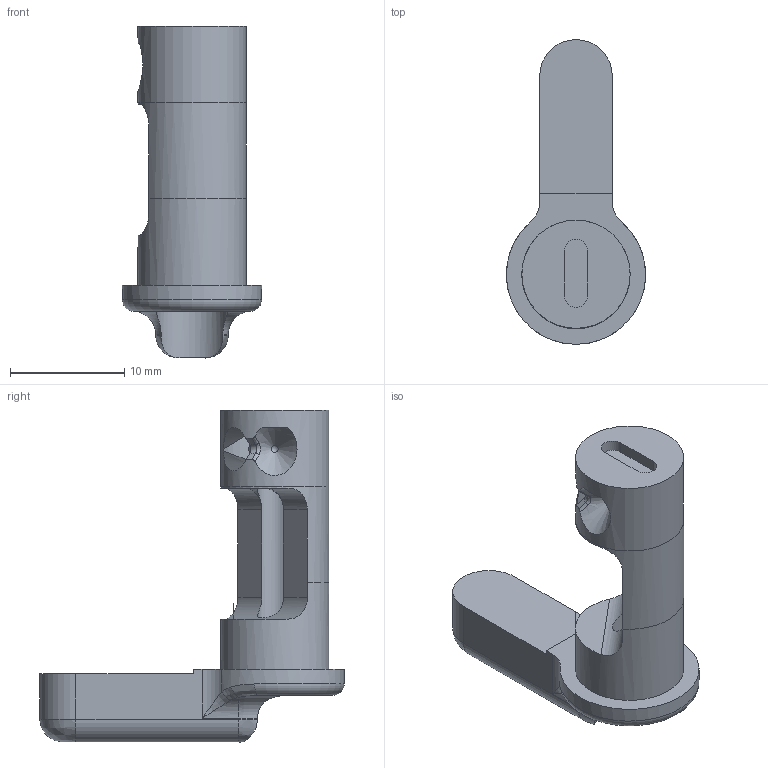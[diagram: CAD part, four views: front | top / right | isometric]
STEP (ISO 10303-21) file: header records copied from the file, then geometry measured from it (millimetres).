
FILE_DESCRIPTION(/* description */ (''),/* implementation_level */ '2;1');
FILE_NAME(/* name */ 'Fire Selector Lever.step',/* time_stamp */ '2022-05-12T09:38:32-06:00',/* author */ (''),/* organization */ (''),/* preprocessor_version */ 'ST-DEVELOPER v18.1',/* originating_system */ 'Autodesk Translation Framework v10.10.0.1391',/* authorisation */ '');
FILE_SCHEMA (('AUTOMOTIVE_DESIGN { 1 0 10303 214 3 1 1 }'));
Length unit declared in the file: millimetre
Products named in the file (1): Fire Selector Lever and drum.
Bounding box: 12.19 x 26.67 x 29.06 mm (x, y, z)
Volume: 1920.6 mm3; surface area: 1544.1 mm2
Topology: 1 solids, 2 shells, 79 faces, 210 edges, 135 vertices
Faces by surface type: plane 29, cylinder 26, bspline 14, cone 4, torus 4, sphere 2
Full cylindrical faces by diameter (mm): 2.87 x1, 3 x1, 9.474 x3
Entity records: 3027 total; most frequent: CARTESIAN_POINT 1094, ORIENTED_EDGE 410, DIRECTION 371, EDGE_CURVE 205, AXIS2_PLACEMENT_3D 149, VERTEX_POINT 135, EDGE_LOOP 86, FACE_OUTER_BOUND 79
